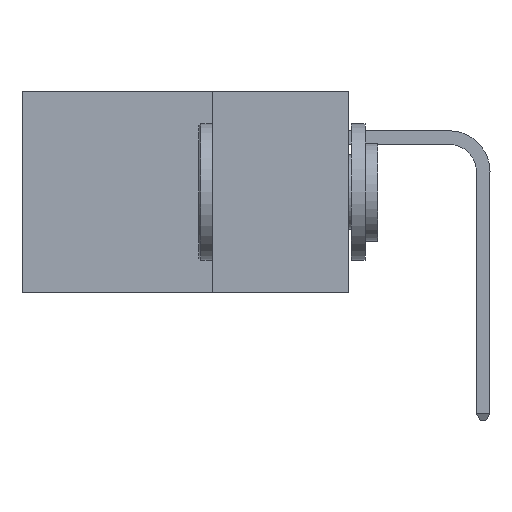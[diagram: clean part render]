
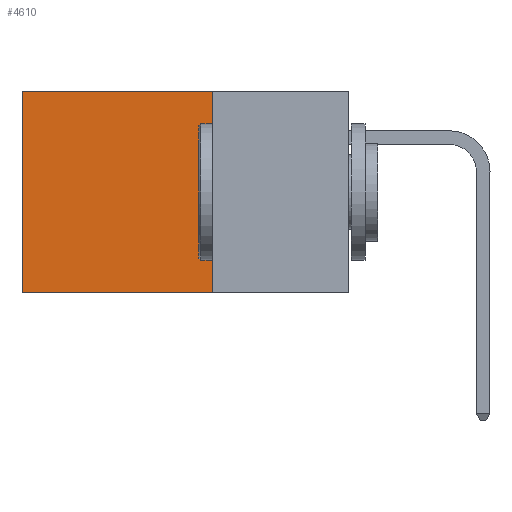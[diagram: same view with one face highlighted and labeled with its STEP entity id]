
A CAD part, left-side view. The second image highlights one B-rep face of the part: STEP entity #4610.
In plain terms, the highlighted planar face has unit normal (-1, 0, 0).
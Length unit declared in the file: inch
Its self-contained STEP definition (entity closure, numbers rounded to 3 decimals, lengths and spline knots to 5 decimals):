
#792 = ORIENTED_EDGE ( 'NONE', *, *, #21114, .F. ) ;
#1528 = ORIENTED_EDGE ( 'NONE', *, *, #13429, .F. ) ;
#1613 = DIRECTION ( 'NONE',  ( 0., 1., 0. ) ) ;
#3092 = VERTEX_POINT ( 'NONE', #35786 ) ;
#3573 = ORIENTED_EDGE ( 'NONE', *, *, #7241, .T. ) ;
#4610 = ADVANCED_FACE ( 'NONE', ( #34624 ), #29355, .F. ) ;
#6926 = CARTESIAN_POINT ( 'NONE',  ( 0.2875, 0.25, -0.37 ) ) ;
#7161 = CARTESIAN_POINT ( 'NONE',  ( 0.2875, 0.6, 0. ) ) ;
#7175 = CARTESIAN_POINT ( 'NONE',  ( 0.2875, 0.6, 0. ) ) ;
#7241 = EDGE_CURVE ( 'NONE', #12639, #3092, #32317, .T. ) ;
#7449 = CARTESIAN_POINT ( 'NONE',  ( 0.2875, 0.25, 0. ) ) ;
#8630 = VERTEX_POINT ( 'NONE', #7449 ) ;
#8756 = LINE ( 'NONE', #10287, #15504 ) ;
#10287 = CARTESIAN_POINT ( 'NONE',  ( 0.2875, 0.25, -0.37 ) ) ;
#12639 = VERTEX_POINT ( 'NONE', #7175 ) ;
#13151 = DIRECTION ( 'NONE',  ( 0., 1., 0. ) ) ;
#13424 = EDGE_CURVE ( 'NONE', #8630, #12639, #17219, .T. ) ;
#13429 = EDGE_CURVE ( 'NONE', #30980, #3092, #8756, .T. ) ;
#14300 = CARTESIAN_POINT ( 'NONE',  ( 0.2875, 0.25, 0. ) ) ;
#15392 = DIRECTION ( 'NONE',  ( 1., 0., 0. ) ) ;
#15504 = VECTOR ( 'NONE', #13151, 39.37008 ) ;
#15815 = DIRECTION ( 'NONE',  ( 0., 0., -1. ) ) ;
#15817 = VECTOR ( 'NONE', #33951, 39.37008 ) ;
#16379 = VECTOR ( 'NONE', #1613, 39.37008 ) ;
#17219 = LINE ( 'NONE', #21540, #16379 ) ;
#21114 = EDGE_CURVE ( 'NONE', #8630, #30980, #29841, .T. ) ;
#21540 = CARTESIAN_POINT ( 'NONE',  ( 0.2875, 0.25, 0. ) ) ;
#21989 = ORIENTED_EDGE ( 'NONE', *, *, #13424, .T. ) ;
#24809 = VECTOR ( 'NONE', #15815, 39.37008 ) ;
#29018 = EDGE_LOOP ( 'NONE', ( #3573, #1528, #792, #21989 ) ) ;
#29355 = PLANE ( 'NONE',  #29697 ) ;
#29697 = AXIS2_PLACEMENT_3D ( 'NONE', #32209, #15392, #35004 ) ;
#29841 = LINE ( 'NONE', #14300, #15817 ) ;
#30980 = VERTEX_POINT ( 'NONE', #6926 ) ;
#32209 = CARTESIAN_POINT ( 'NONE',  ( 0.2875, 0.25, 0. ) ) ;
#32317 = LINE ( 'NONE', #7161, #24809 ) ;
#33951 = DIRECTION ( 'NONE',  ( 0., 0., -1. ) ) ;
#34624 = FACE_OUTER_BOUND ( 'NONE', #29018, .T. ) ;
#35004 = DIRECTION ( 'NONE',  ( 0., 0., -1. ) ) ;
#35786 = CARTESIAN_POINT ( 'NONE',  ( 0.2875, 0.6, -0.37 ) ) ;
